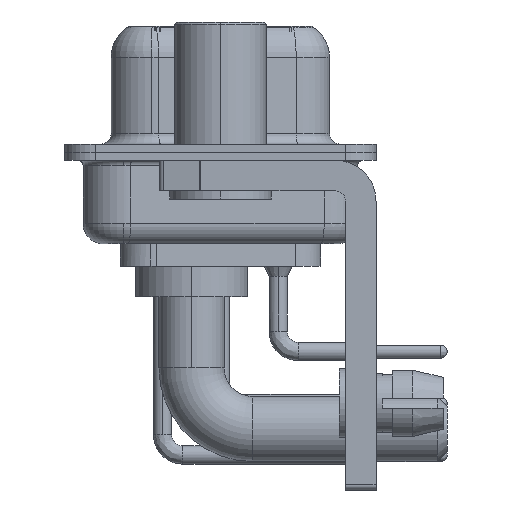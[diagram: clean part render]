
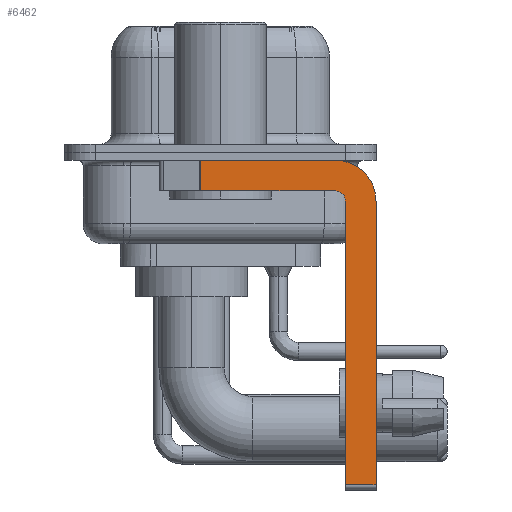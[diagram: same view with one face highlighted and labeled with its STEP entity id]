
A CAD part, left-side view. The second image highlights one B-rep face of the part: STEP entity #6462.
In plain terms, the highlighted planar face has unit normal (-1, 0, 0).
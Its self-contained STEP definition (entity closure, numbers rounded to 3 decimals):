
#387 = VECTOR ( 'NONE', #26058, 1000. ) ;
#1909 = DIRECTION ( 'NONE',  ( 0., 0., 1. ) ) ;
#1973 = VECTOR ( 'NONE', #22381, 1000. ) ;
#2598 = EDGE_CURVE ( 'NONE', #23532, #9088, #31862, .T. ) ;
#2787 = EDGE_CURVE ( 'NONE', #3627, #24989, #17278, .T. ) ;
#2831 = FACE_OUTER_BOUND ( 'NONE', #19054, .T. ) ;
#3627 = VERTEX_POINT ( 'NONE', #27821 ) ;
#3723 = ORIENTED_EDGE ( 'NONE', *, *, #11124, .T. ) ;
#4123 = CARTESIAN_POINT ( 'NONE',  ( -2.9, -7.65, -2.4 ) ) ;
#5371 = CARTESIAN_POINT ( 'NONE',  ( -2.9, -5.65, -2.4 ) ) ;
#5637 = AXIS2_PLACEMENT_3D ( 'NONE', #5371, #8398, #13473 ) ;
#5656 = DIRECTION ( 'NONE',  ( 1., 0., 0. ) ) ;
#5805 = VERTEX_POINT ( 'NONE', #11828 ) ;
#6048 = VERTEX_POINT ( 'NONE', #21631 ) ;
#6211 = CARTESIAN_POINT ( 'NONE',  ( -2.9, 0.978, -1.9 ) ) ;
#6462 = ADVANCED_FACE ( 'NONE', ( #2831 ), #16179, .F. ) ;
#6597 = DIRECTION ( 'NONE',  ( 0., 0., 1. ) ) ;
#6977 = CIRCLE ( 'NONE', #25901, 2. ) ;
#7431 = CARTESIAN_POINT ( 'NONE',  ( -2.9, -5.65, -0.4 ) ) ;
#8185 = DIRECTION ( 'NONE',  ( 0., 0., -1. ) ) ;
#8398 = DIRECTION ( 'NONE',  ( 1., 0., 0. ) ) ;
#8408 = CARTESIAN_POINT ( 'NONE',  ( -2.9, -7.65, -16.35 ) ) ;
#9088 = VERTEX_POINT ( 'NONE', #7431 ) ;
#10162 = VECTOR ( 'NONE', #15749, 1000. ) ;
#10360 = EDGE_CURVE ( 'NONE', #5805, #19985, #22710, .T. ) ;
#10448 = EDGE_CURVE ( 'NONE', #6048, #3627, #20894, .T. ) ;
#10613 = CARTESIAN_POINT ( 'NONE',  ( -2.9, 0.978, -0.4 ) ) ;
#10968 = CARTESIAN_POINT ( 'NONE',  ( -2.9, -5.65, -16.35 ) ) ;
#11124 = EDGE_CURVE ( 'NONE', #13902, #19985, #31966, .T. ) ;
#11438 = VECTOR ( 'NONE', #23741, 1000. ) ;
#11828 = CARTESIAN_POINT ( 'NONE',  ( -2.9, -7.65, -2.4 ) ) ;
#13473 = DIRECTION ( 'NONE',  ( 0., 0., -1. ) ) ;
#13701 = CARTESIAN_POINT ( 'NONE',  ( -2.9, 0.978, -1.9 ) ) ;
#13902 = VERTEX_POINT ( 'NONE', #22887 ) ;
#14073 = CARTESIAN_POINT ( 'NONE',  ( -2.9, -5.65, -1.9 ) ) ;
#15224 = ORIENTED_EDGE ( 'NONE', *, *, #31754, .F. ) ;
#15749 = DIRECTION ( 'NONE',  ( 0., 0., -1. ) ) ;
#15790 = CARTESIAN_POINT ( 'NONE',  ( -2.9, 3., -0.4 ) ) ;
#16179 = PLANE ( 'NONE',  #5637 ) ;
#16960 = CARTESIAN_POINT ( 'NONE',  ( -2.9, -5.65, -2.4 ) ) ;
#17278 = LINE ( 'NONE', #14073, #22845 ) ;
#17681 = ORIENTED_EDGE ( 'NONE', *, *, #27194, .T. ) ;
#18756 = ORIENTED_EDGE ( 'NONE', *, *, #33303, .F. ) ;
#18834 = CARTESIAN_POINT ( 'NONE',  ( -2.9, -6.15, -16.6 ) ) ;
#18838 = ORIENTED_EDGE ( 'NONE', *, *, #10448, .F. ) ;
#19054 = EDGE_LOOP ( 'NONE', ( #21049, #17681, #29127, #18838, #18756, #3723, #26703, #15224 ) ) ;
#19985 = VERTEX_POINT ( 'NONE', #8408 ) ;
#20894 = CIRCLE ( 'NONE', #29558, 0.5 ) ;
#21049 = ORIENTED_EDGE ( 'NONE', *, *, #2598, .F. ) ;
#21631 = CARTESIAN_POINT ( 'NONE',  ( -2.9, -6.15, -2.4 ) ) ;
#22381 = DIRECTION ( 'NONE',  ( 0., 0., -1. ) ) ;
#22710 = LINE ( 'NONE', #4123, #1973 ) ;
#22845 = VECTOR ( 'NONE', #27283, 1000. ) ;
#22887 = CARTESIAN_POINT ( 'NONE',  ( -2.9, -6.15, -16.35 ) ) ;
#23532 = VERTEX_POINT ( 'NONE', #10613 ) ;
#23741 = DIRECTION ( 'NONE',  ( 0., -1., 0. ) ) ;
#24989 = VERTEX_POINT ( 'NONE', #6211 ) ;
#25372 = VECTOR ( 'NONE', #6597, 1000. ) ;
#25901 = AXIS2_PLACEMENT_3D ( 'NONE', #28846, #5656, #8185 ) ;
#26058 = DIRECTION ( 'NONE',  ( 0., -1., 0. ) ) ;
#26703 = ORIENTED_EDGE ( 'NONE', *, *, #10360, .F. ) ;
#27194 = EDGE_CURVE ( 'NONE', #23532, #24989, #31336, .T. ) ;
#27283 = DIRECTION ( 'NONE',  ( 0., 1., 0. ) ) ;
#27821 = CARTESIAN_POINT ( 'NONE',  ( -2.9, -5.65, -1.9 ) ) ;
#28846 = CARTESIAN_POINT ( 'NONE',  ( -2.9, -5.65, -2.4 ) ) ;
#29127 = ORIENTED_EDGE ( 'NONE', *, *, #2787, .F. ) ;
#29558 = AXIS2_PLACEMENT_3D ( 'NONE', #16960, #32720, #1909 ) ;
#31336 = LINE ( 'NONE', #13701, #10162 ) ;
#31711 = LINE ( 'NONE', #18834, #25372 ) ;
#31754 = EDGE_CURVE ( 'NONE', #9088, #5805, #6977, .T. ) ;
#31862 = LINE ( 'NONE', #15790, #11438 ) ;
#31966 = LINE ( 'NONE', #10968, #387 ) ;
#32720 = DIRECTION ( 'NONE',  ( -1., 0., 0. ) ) ;
#33303 = EDGE_CURVE ( 'NONE', #13902, #6048, #31711, .T. ) ;
